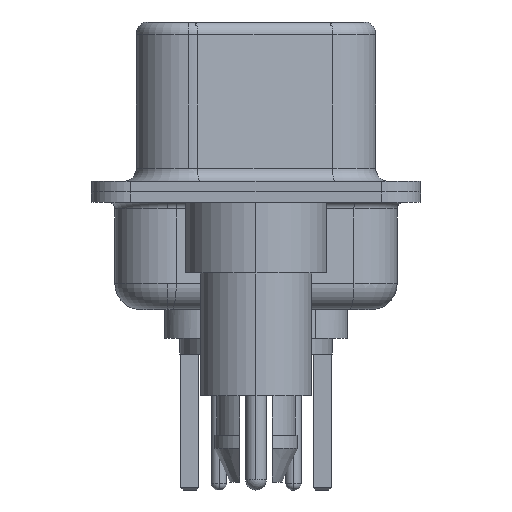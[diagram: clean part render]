
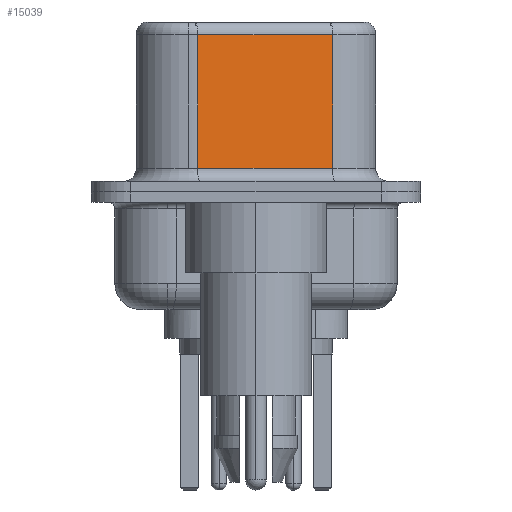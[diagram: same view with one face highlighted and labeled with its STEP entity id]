
A CAD part, left-side view. The second image highlights one B-rep face of the part: STEP entity #15039.
In plain terms, the highlighted planar face has unit normal (-0.985, -0.174, 0).
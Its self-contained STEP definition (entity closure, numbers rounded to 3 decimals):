
#12 = CARTESIAN_POINT ( 'NONE',  ( 4.58, -2.927, 0.9 ) ) ;
#1151 = AXIS2_PLACEMENT_3D ( 'NONE', #22866, #11315, #24755 ) ;
#5125 = CARTESIAN_POINT ( 'NONE',  ( 4.58, -2.927, 0.9 ) ) ;
#6821 = VERTEX_POINT ( 'NONE', #19263 ) ;
#6884 = FACE_OUTER_BOUND ( 'NONE', #8974, .T. ) ;
#7072 = DIRECTION ( 'NONE',  ( 0.174, -0.985, 0. ) ) ;
#8900 = VERTEX_POINT ( 'NONE', #15023 ) ;
#8974 = EDGE_LOOP ( 'NONE', ( #20801, #15330, #18363, #16837 ) ) ;
#9357 = PLANE ( 'NONE',  #1151 ) ;
#9542 = DIRECTION ( 'NONE',  ( -0.174, 0.985, 0. ) ) ;
#11315 = DIRECTION ( 'NONE',  ( 0.985, 0.174, 0. ) ) ;
#11606 = DIRECTION ( 'NONE',  ( 0., 0., -1. ) ) ;
#11939 = LINE ( 'NONE', #17199, #22199 ) ;
#12450 = DIRECTION ( 'NONE',  ( 0., 0., -1. ) ) ;
#13122 = VECTOR ( 'NONE', #11606, 1000. ) ;
#14800 = EDGE_CURVE ( 'NONE', #23983, #6821, #21049, .T. ) ;
#15023 = CARTESIAN_POINT ( 'NONE',  ( 4.58, -2.927, 6.02 ) ) ;
#15039 = ADVANCED_FACE ( 'NONE', ( #6884 ), #9357, .F. ) ;
#15330 = ORIENTED_EDGE ( 'NONE', *, *, #16602, .T. ) ;
#16602 = EDGE_CURVE ( 'NONE', #8900, #23983, #11939, .T. ) ;
#16837 = ORIENTED_EDGE ( 'NONE', *, *, #20322, .T. ) ;
#17053 = CARTESIAN_POINT ( 'NONE',  ( 3.67, 2.233, 6.02 ) ) ;
#17078 = VECTOR ( 'NONE', #12450, 1000. ) ;
#17199 = CARTESIAN_POINT ( 'NONE',  ( 4.58, -2.927, 6.02 ) ) ;
#17824 = EDGE_CURVE ( 'NONE', #8900, #21652, #18207, .T. ) ;
#17825 = VECTOR ( 'NONE', #7072, 1000. ) ;
#18207 = LINE ( 'NONE', #23142, #13122 ) ;
#18363 = ORIENTED_EDGE ( 'NONE', *, *, #14800, .T. ) ;
#18455 = LINE ( 'NONE', #5125, #17825 ) ;
#19263 = CARTESIAN_POINT ( 'NONE',  ( 3.67, 2.233, 0.9 ) ) ;
#20322 = EDGE_CURVE ( 'NONE', #6821, #21652, #18455, .T. ) ;
#20801 = ORIENTED_EDGE ( 'NONE', *, *, #17824, .F. ) ;
#21049 = LINE ( 'NONE', #23928, #17078 ) ;
#21652 = VERTEX_POINT ( 'NONE', #12 ) ;
#22199 = VECTOR ( 'NONE', #9542, 1000. ) ;
#22866 = CARTESIAN_POINT ( 'NONE',  ( 4.58, -2.927, 6.52 ) ) ;
#23142 = CARTESIAN_POINT ( 'NONE',  ( 4.58, -2.927, 6.52 ) ) ;
#23928 = CARTESIAN_POINT ( 'NONE',  ( 3.67, 2.233, 6.52 ) ) ;
#23983 = VERTEX_POINT ( 'NONE', #17053 ) ;
#24755 = DIRECTION ( 'NONE',  ( -0.174, 0.985, 0. ) ) ;
